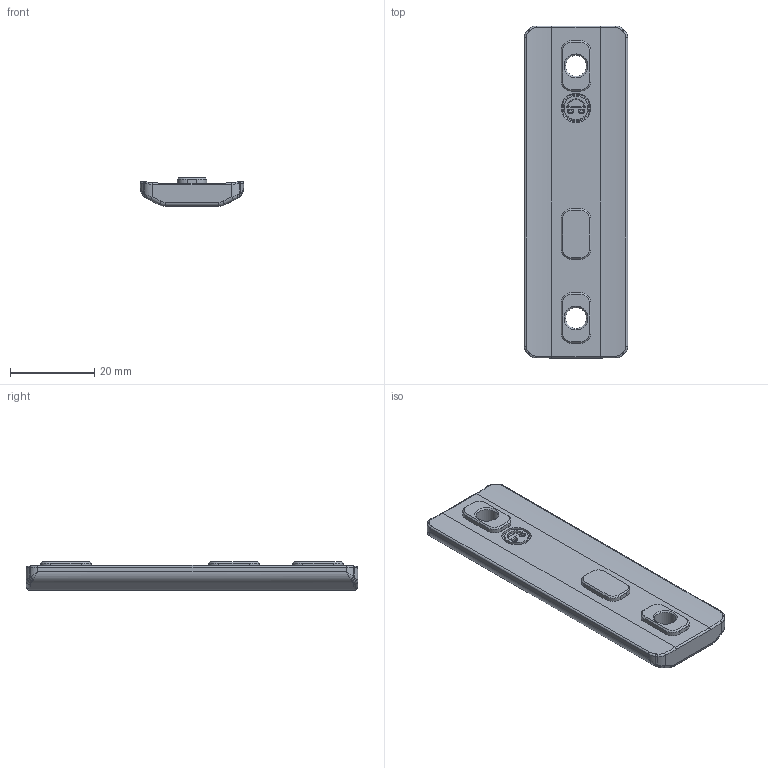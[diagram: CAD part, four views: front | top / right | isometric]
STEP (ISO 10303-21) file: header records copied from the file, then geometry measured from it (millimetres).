
FILE_DESCRIPTION(/* description */ (''),/* implementation_level */ '2;1');
FILE_NAME(/* name */ '2 Slot.step',/* time_stamp */ '2021-09-29T15:51:47-04:00',/* author */ (''),/* organization */ (''),/* preprocessor_version */ 'ST-DEVELOPER v18.1',/* originating_system */ 'Autodesk Translation Framework v10.10.0.1391',/* authorisation */ '');
FILE_SCHEMA (('AUTOMOTIVE_DESIGN { 1 0 10303 214 3 1 1 }'));
Length unit declared in the file: millimetre
Products named in the file (1): 2 Slot
Bounding box: 24.6 x 79 x 6.85 mm (x, y, z)
Volume: 9421.9 mm3; surface area: 4944.9 mm2
Topology: 1 solids, 1 shells, 166 faces, 377 edges, 219 vertices
Faces by surface type: cylinder 54, plane 46, bspline 30, torus 16, cone 16, sphere 4
Full cylindrical faces by diameter (mm): 5 x2, 5.6 x1, 7 x1, 9.3 x2
Entity records: 5174 total; most frequent: CARTESIAN_POINT 1459, DIRECTION 796, ORIENTED_EDGE 746, EDGE_CURVE 373, AXIS2_PLACEMENT_3D 322, VERTEX_POINT 219, EDGE_LOOP 180, FACE_OUTER_BOUND 166
